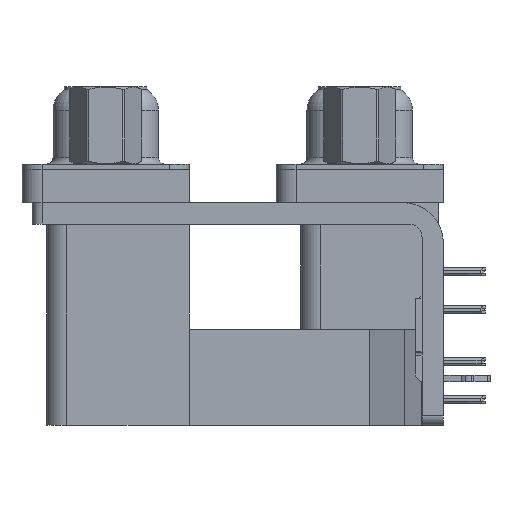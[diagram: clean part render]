
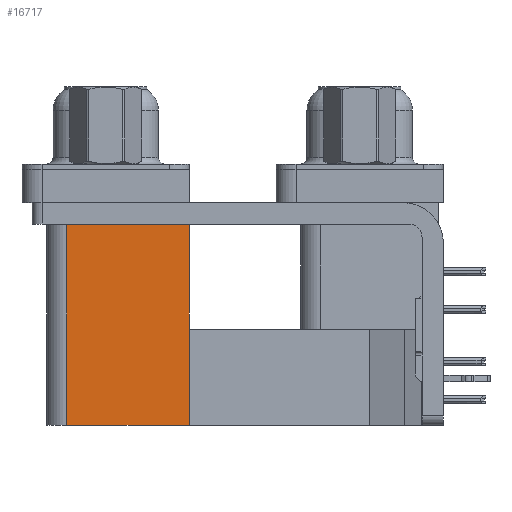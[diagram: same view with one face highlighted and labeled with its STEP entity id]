
A CAD part, left-side view. The second image highlights one B-rep face of the part: STEP entity #16717.
In plain terms, the highlighted planar face has unit normal (-1, 0, 0).
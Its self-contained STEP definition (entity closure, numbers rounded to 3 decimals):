
#1127 = DIRECTION ( 'NONE',  ( 0., 0., 1. ) ) ;
#2405 = VERTEX_POINT ( 'NONE', #27820 ) ;
#2651 = FACE_OUTER_BOUND ( 'NONE', #6485, .T. ) ;
#4136 = CARTESIAN_POINT ( 'NONE',  ( 3.79, 21.975, -19.2 ) ) ;
#5886 = PLANE ( 'NONE',  #14405 ) ;
#6485 = EDGE_LOOP ( 'NONE', ( #47984, #16028, #25803, #41754 ) ) ;
#8370 = CARTESIAN_POINT ( 'NONE',  ( 3.79, 21.975, -2.5 ) ) ;
#8592 = EDGE_CURVE ( 'NONE', #46425, #33288, #31181, .T. ) ;
#11752 = DIRECTION ( 'NONE',  ( 0., 0., 1. ) ) ;
#12247 = CARTESIAN_POINT ( 'NONE',  ( 3.79, 12.775, -19.2 ) ) ;
#14405 = AXIS2_PLACEMENT_3D ( 'NONE', #25796, #33201, #36440 ) ;
#15177 = LINE ( 'NONE', #30175, #46905 ) ;
#15905 = CARTESIAN_POINT ( 'NONE',  ( 3.79, 12.775, -19.2 ) ) ;
#16028 = ORIENTED_EDGE ( 'NONE', *, *, #8592, .F. ) ;
#16717 = ADVANCED_FACE ( 'NONE', ( #2651 ), #5886, .F. ) ;
#19885 = CARTESIAN_POINT ( 'NONE',  ( 3.79, 21.975, -19.2 ) ) ;
#19906 = LINE ( 'NONE', #31456, #23232 ) ;
#23232 = VECTOR ( 'NONE', #38385, 1000. ) ;
#25796 = CARTESIAN_POINT ( 'NONE',  ( 3.79, 12.775, -19.2 ) ) ;
#25803 = ORIENTED_EDGE ( 'NONE', *, *, #26855, .F. ) ;
#25830 = EDGE_CURVE ( 'NONE', #27339, #2405, #30964, .T. ) ;
#26855 = EDGE_CURVE ( 'NONE', #27339, #46425, #19906, .T. ) ;
#27208 = EDGE_CURVE ( 'NONE', #2405, #33288, #15177, .T. ) ;
#27339 = VERTEX_POINT ( 'NONE', #15905 ) ;
#27820 = CARTESIAN_POINT ( 'NONE',  ( 3.79, 12.775, -2.5 ) ) ;
#30175 = CARTESIAN_POINT ( 'NONE',  ( 3.79, 12.775, -2.5 ) ) ;
#30964 = LINE ( 'NONE', #12247, #48355 ) ;
#31181 = LINE ( 'NONE', #19885, #44759 ) ;
#31456 = CARTESIAN_POINT ( 'NONE',  ( 3.79, 12.775, -19.2 ) ) ;
#33201 = DIRECTION ( 'NONE',  ( 1., 0., 0. ) ) ;
#33288 = VERTEX_POINT ( 'NONE', #8370 ) ;
#36440 = DIRECTION ( 'NONE',  ( 0., 1., 0. ) ) ;
#38385 = DIRECTION ( 'NONE',  ( 0., 1., 0. ) ) ;
#41754 = ORIENTED_EDGE ( 'NONE', *, *, #25830, .T. ) ;
#44759 = VECTOR ( 'NONE', #1127, 1000. ) ;
#45237 = DIRECTION ( 'NONE',  ( 0., 1., 0. ) ) ;
#46425 = VERTEX_POINT ( 'NONE', #4136 ) ;
#46905 = VECTOR ( 'NONE', #45237, 1000. ) ;
#47984 = ORIENTED_EDGE ( 'NONE', *, *, #27208, .T. ) ;
#48355 = VECTOR ( 'NONE', #11752, 1000. ) ;
